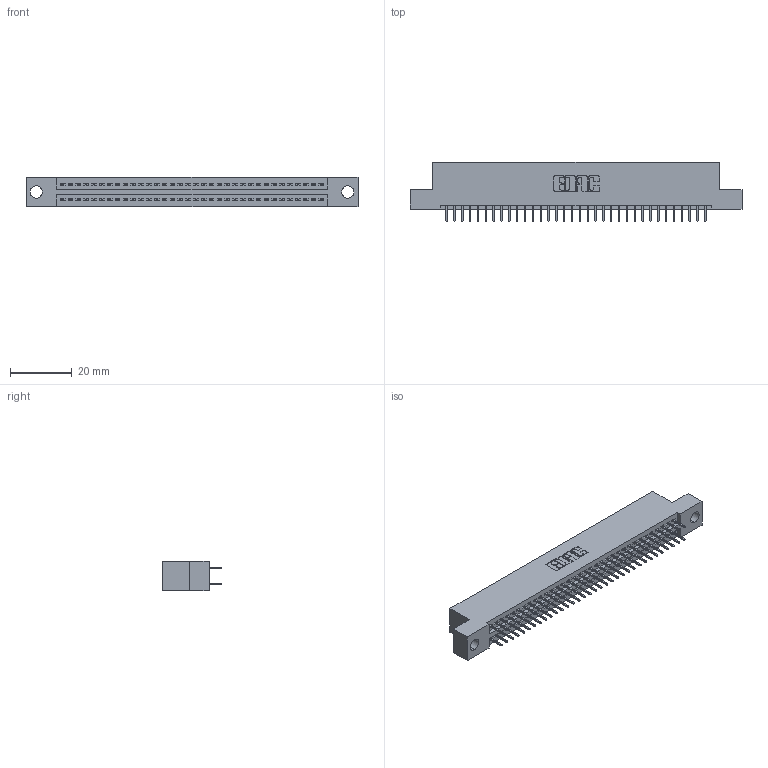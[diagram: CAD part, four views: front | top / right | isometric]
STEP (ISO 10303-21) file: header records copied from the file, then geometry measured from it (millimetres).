
FILE_DESCRIPTION (( 'STEP AP203' ), '1' );
FILE_NAME ('395-068-524-204.STEP', '2021-06-17T03:53:28', ( '' ), ( '' ), 'SwSTEP 2.0', 'SolidWorks 2020', '' );
FILE_SCHEMA (( 'CONFIG_CONTROL_DESIGN' ));
Length unit declared in the file: inch
Products named in the file (3): 345 Part_Flush Mounting Lugs - 0.156 Dia-TI; 395-068-524-204; 345-292-001_345-293-124
Assembly tree (69 placements, depth 2):
  395-068-524-204
    345 Part_Flush Mounting Lugs - 0.156 Dia-TI
    345-292-001_345-293-124  x68
Bounding box: 107.57 x 19.35 x 9.4 mm (x, y, z)
Volume: 10166.2 mm3; surface area: 14452.4 mm2
Topology: 69 solids, 69 shells, 3812 faces, 10781 edges, 6914 vertices
Faces by surface type: plane 2746, cylinder 1066
Entity records: 28247 total; most frequent: CARTESIAN_POINT 4746, ORIENTED_EDGE 4678, DIRECTION 4195, EDGE_CURVE 2339, LINE 2075, VECTOR 2075, VERTEX_POINT 1554, AXIS2_PLACEMENT_3D 1060
